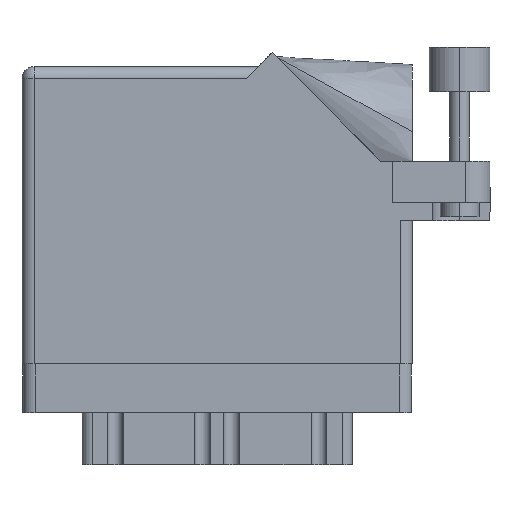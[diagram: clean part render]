
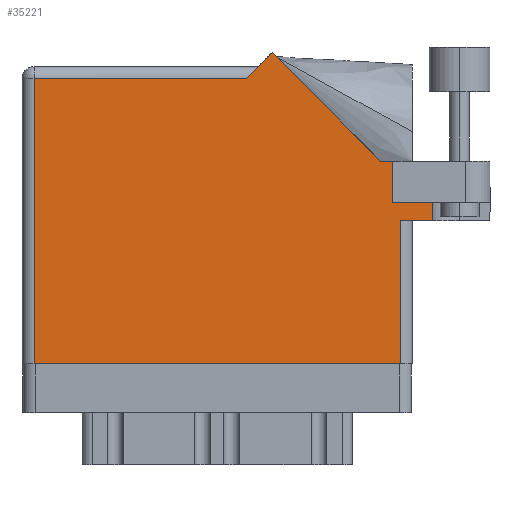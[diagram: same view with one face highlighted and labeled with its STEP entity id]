
A CAD part, front view. The second image highlights one B-rep face of the part: STEP entity #35221.
In plain terms, the highlighted face is planar.
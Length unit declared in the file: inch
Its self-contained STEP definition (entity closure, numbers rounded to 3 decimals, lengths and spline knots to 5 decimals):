
#824 = ORIENTED_EDGE ( 'NONE', *, *, #7759, .T. ) ;
#1579 = AXIS2_PLACEMENT_3D ( 'NONE', #30254, #3060, #21725 ) ;
#1671 = LINE ( 'NONE', #35355, #7833 ) ;
#3060 = DIRECTION ( 'NONE',  ( 0., 0., -1. ) ) ;
#3259 = LINE ( 'NONE', #24699, #37208 ) ;
#3453 = CARTESIAN_POINT ( 'NONE',  ( 1.948, 0., 0. ) ) ;
#3713 = VERTEX_POINT ( 'NONE', #30703 ) ;
#3964 = DIRECTION ( 'NONE',  ( -1., 0., 0. ) ) ;
#5144 = VERTEX_POINT ( 'NONE', #32092 ) ;
#6436 = VECTOR ( 'NONE', #37520, 39.37008 ) ;
#6545 = ORIENTED_EDGE ( 'NONE', *, *, #23336, .T. ) ;
#7759 = EDGE_CURVE ( 'NONE', #20781, #32137, #28007, .T. ) ;
#7833 = VECTOR ( 'NONE', #34767, 39.37008 ) ;
#8554 = CARTESIAN_POINT ( 'NONE',  ( 2.1115, 1.16177, 0. ) ) ;
#9033 = LINE ( 'NONE', #35996, #36774 ) ;
#9403 = FACE_OUTER_BOUND ( 'NONE', #36737, .T. ) ;
#10457 = CARTESIAN_POINT ( 'NONE',  ( 1.948, 0.737, 0. ) ) ;
#10686 = VECTOR ( 'NONE', #22058, 39.37008 ) ;
#10898 = DIRECTION ( 'NONE',  ( -0.707, -0.707, 0. ) ) ;
#11574 = CARTESIAN_POINT ( 'NONE',  ( 2.1115, 0.831, 0. ) ) ;
#12162 = CARTESIAN_POINT ( 'NONE',  ( 1.84442, 1.044, 0. ) ) ;
#12503 = CARTESIAN_POINT ( 'NONE',  ( 1.91, 1.044, 0. ) ) ;
#12918 = LINE ( 'NONE', #19067, #21452 ) ;
#13243 = LINE ( 'NONE', #10457, #31042 ) ;
#14643 = EDGE_CURVE ( 'NONE', #29883, #5144, #35717, .T. ) ;
#14919 = DIRECTION ( 'NONE',  ( 0., -1., 0. ) ) ;
#14938 = EDGE_CURVE ( 'NONE', #38345, #36512, #34881, .T. ) ;
#15507 = ORIENTED_EDGE ( 'NONE', *, *, #32485, .T. ) ;
#15663 = EDGE_CURVE ( 'NONE', #22350, #29883, #3259, .T. ) ;
#15833 = DIRECTION ( 'NONE',  ( 0., 1., 0. ) ) ;
#16325 = LINE ( 'NONE', #39172, #10686 ) ;
#16854 = ORIENTED_EDGE ( 'NONE', *, *, #38264, .T. ) ;
#19067 = CARTESIAN_POINT ( 'NONE',  ( 0., 1.468, 0. ) ) ;
#19144 = CARTESIAN_POINT ( 'NONE',  ( 1.91, 0.831, 0. ) ) ;
#19502 = DIRECTION ( 'NONE',  ( 1., 0., 0. ) ) ;
#20568 = LINE ( 'NONE', #23924, #22198 ) ;
#20781 = VERTEX_POINT ( 'NONE', #12503 ) ;
#20782 = VECTOR ( 'NONE', #14919, 39.37008 ) ;
#21098 = DIRECTION ( 'NONE',  ( -0.707, 0.707, 0. ) ) ;
#21452 = VECTOR ( 'NONE', #3964, 39.37008 ) ;
#21725 = DIRECTION ( 'NONE',  ( -1., 0., 0. ) ) ;
#22058 = DIRECTION ( 'NONE',  ( 0., 1., 0. ) ) ;
#22198 = VECTOR ( 'NONE', #32649, 39.37008 ) ;
#22350 = VERTEX_POINT ( 'NONE', #19144 ) ;
#22383 = CARTESIAN_POINT ( 'NONE',  ( 0.062, 1.468, 0. ) ) ;
#22640 = ORIENTED_EDGE ( 'NONE', *, *, #15663, .F. ) ;
#23230 = VECTOR ( 'NONE', #21098, 39.37008 ) ;
#23336 = EDGE_CURVE ( 'NONE', #32137, #38345, #27236, .T. ) ;
#23871 = VECTOR ( 'NONE', #10898, 39.37008 ) ;
#23924 = CARTESIAN_POINT ( 'NONE',  ( 0.062, 0., 0. ) ) ;
#24246 = VERTEX_POINT ( 'NONE', #22383 ) ;
#24699 = CARTESIAN_POINT ( 'NONE',  ( 1.91, 0.831, 0. ) ) ;
#24775 = VERTEX_POINT ( 'NONE', #34406 ) ;
#24898 = PLANE ( 'NONE',  #1579 ) ;
#25214 = EDGE_CURVE ( 'NONE', #36512, #24246, #12918, .T. ) ;
#25418 = CARTESIAN_POINT ( 'NONE',  ( 2.41, 1.044, 0. ) ) ;
#26918 = ORIENTED_EDGE ( 'NONE', *, *, #36922, .T. ) ;
#27125 = EDGE_CURVE ( 'NONE', #22350, #20781, #16325, .T. ) ;
#27236 = LINE ( 'NONE', #12162, #23230 ) ;
#28007 = LINE ( 'NONE', #25418, #6436 ) ;
#28096 = ORIENTED_EDGE ( 'NONE', *, *, #25214, .T. ) ;
#28476 = VERTEX_POINT ( 'NONE', #3453 ) ;
#28963 = CARTESIAN_POINT ( 'NONE',  ( 1.217, 1.53, 0. ) ) ;
#29093 = CARTESIAN_POINT ( 'NONE',  ( 1.84442, 1.044, 0. ) ) ;
#29811 = ORIENTED_EDGE ( 'NONE', *, *, #14643, .F. ) ;
#29883 = VERTEX_POINT ( 'NONE', #11574 ) ;
#30254 = CARTESIAN_POINT ( 'NONE',  ( 0., 1.53, 0. ) ) ;
#30290 = CARTESIAN_POINT ( 'NONE',  ( 1.155, 1.468, 0. ) ) ;
#30703 = CARTESIAN_POINT ( 'NONE',  ( 1.948, 0.737, 0. ) ) ;
#31042 = VECTOR ( 'NONE', #15833, 39.37008 ) ;
#31363 = ORIENTED_EDGE ( 'NONE', *, *, #27125, .T. ) ;
#32092 = CARTESIAN_POINT ( 'NONE',  ( 2.1115, 0.737, 0. ) ) ;
#32137 = VERTEX_POINT ( 'NONE', #29093 ) ;
#32485 = EDGE_CURVE ( 'NONE', #3713, #5144, #1671, .T. ) ;
#32649 = DIRECTION ( 'NONE',  ( 0., -1., 0. ) ) ;
#32843 = DIRECTION ( 'NONE',  ( 1., 0., 0. ) ) ;
#34406 = CARTESIAN_POINT ( 'NONE',  ( 0.062, 0., 0. ) ) ;
#34767 = DIRECTION ( 'NONE',  ( 1., 0., 0. ) ) ;
#34881 = LINE ( 'NONE', #28963, #23871 ) ;
#35221 = ADVANCED_FACE ( 'NONE', ( #9403 ), #24898, .F. ) ;
#35355 = CARTESIAN_POINT ( 'NONE',  ( 2.01, 0.737, 0. ) ) ;
#35717 = LINE ( 'NONE', #8554, #20782 ) ;
#35996 = CARTESIAN_POINT ( 'NONE',  ( 0., 0., 0. ) ) ;
#36512 = VERTEX_POINT ( 'NONE', #30290 ) ;
#36737 = EDGE_LOOP ( 'NONE', ( #16854, #37851, #15507, #29811, #22640, #31363, #824, #6545, #38956, #28096, #26918 ) ) ;
#36774 = VECTOR ( 'NONE', #32843, 39.37008 ) ;
#36922 = EDGE_CURVE ( 'NONE', #24246, #24775, #20568, .T. ) ;
#37208 = VECTOR ( 'NONE', #19502, 39.37008 ) ;
#37520 = DIRECTION ( 'NONE',  ( -1., 0., 0. ) ) ;
#37851 = ORIENTED_EDGE ( 'NONE', *, *, #38623, .T. ) ;
#38137 = CARTESIAN_POINT ( 'NONE',  ( 1.28771, 1.60071, 0. ) ) ;
#38264 = EDGE_CURVE ( 'NONE', #24775, #28476, #9033, .T. ) ;
#38345 = VERTEX_POINT ( 'NONE', #38137 ) ;
#38623 = EDGE_CURVE ( 'NONE', #28476, #3713, #13243, .T. ) ;
#38956 = ORIENTED_EDGE ( 'NONE', *, *, #14938, .T. ) ;
#39172 = CARTESIAN_POINT ( 'NONE',  ( 1.91, 0.831, 0. ) ) ;
